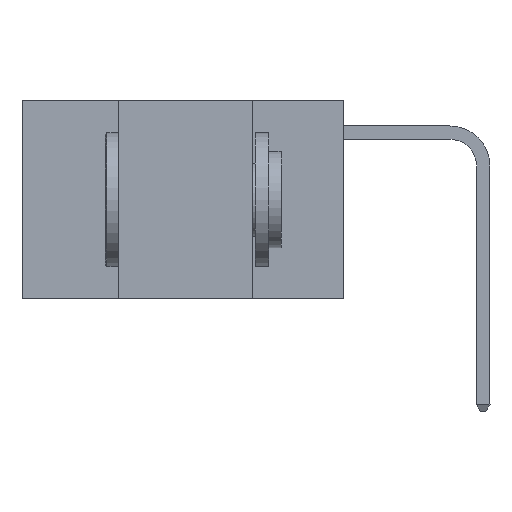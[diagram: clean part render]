
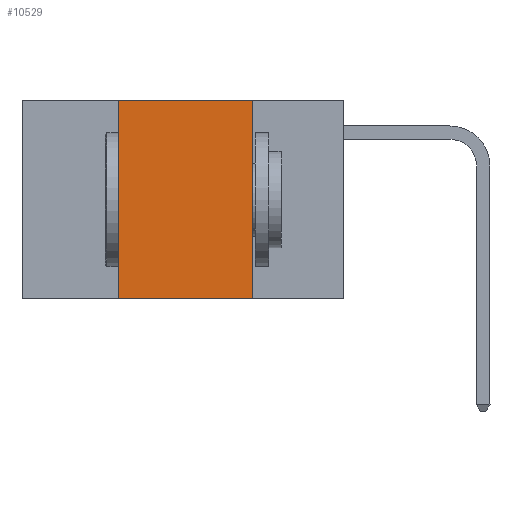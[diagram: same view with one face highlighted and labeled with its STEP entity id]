
A CAD part, left-side view. The second image highlights one B-rep face of the part: STEP entity #10529.
In plain terms, the highlighted planar face has unit normal (-1, 0, 0).
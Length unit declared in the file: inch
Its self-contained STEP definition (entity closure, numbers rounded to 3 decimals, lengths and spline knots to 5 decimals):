
#211 = CARTESIAN_POINT ( 'NONE',  ( 0., 0.42, -0.37 ) ) ;
#345 = PLANE ( 'NONE',  #6975 ) ;
#866 = CARTESIAN_POINT ( 'NONE',  ( 0., 0.17, -0.37 ) ) ;
#895 = VECTOR ( 'NONE', #1510, 39.37008 ) ;
#990 = ORIENTED_EDGE ( 'NONE', *, *, #8461, .F. ) ;
#1510 = DIRECTION ( 'NONE',  ( 0., 0., 1. ) ) ;
#1576 = EDGE_CURVE ( 'NONE', #8686, #7853, #7452, .T. ) ;
#1578 = DIRECTION ( 'NONE',  ( 0., 0., -1. ) ) ;
#1854 = VECTOR ( 'NONE', #11834, 39.37008 ) ;
#2192 = LINE ( 'NONE', #7042, #10957 ) ;
#3244 = FACE_OUTER_BOUND ( 'NONE', #6605, .T. ) ;
#4313 = ORIENTED_EDGE ( 'NONE', *, *, #9309, .T. ) ;
#4611 = ORIENTED_EDGE ( 'NONE', *, *, #1576, .F. ) ;
#5503 = VERTEX_POINT ( 'NONE', #866 ) ;
#6434 = DIRECTION ( 'NONE',  ( 0., 0., -1. ) ) ;
#6499 = LINE ( 'NONE', #10439, #10094 ) ;
#6605 = EDGE_LOOP ( 'NONE', ( #990, #7960, #4611, #4313 ) ) ;
#6975 = AXIS2_PLACEMENT_3D ( 'NONE', #9338, #9401, #6434 ) ;
#7042 = CARTESIAN_POINT ( 'NONE',  ( 0., 0.6, 0. ) ) ;
#7452 = LINE ( 'NONE', #10370, #895 ) ;
#7853 = VERTEX_POINT ( 'NONE', #9164 ) ;
#7879 = CARTESIAN_POINT ( 'NONE',  ( 0., 0.6, -0.37 ) ) ;
#7960 = ORIENTED_EDGE ( 'NONE', *, *, #11974, .F. ) ;
#8461 = EDGE_CURVE ( 'NONE', #9494, #5503, #6499, .T. ) ;
#8686 = VERTEX_POINT ( 'NONE', #211 ) ;
#9164 = CARTESIAN_POINT ( 'NONE',  ( 0., 0.42, 0. ) ) ;
#9309 = EDGE_CURVE ( 'NONE', #8686, #5503, #11708, .T. ) ;
#9338 = CARTESIAN_POINT ( 'NONE',  ( 0., 0.6, 0. ) ) ;
#9401 = DIRECTION ( 'NONE',  ( 1., 0., 0. ) ) ;
#9494 = VERTEX_POINT ( 'NONE', #11507 ) ;
#10094 = VECTOR ( 'NONE', #1578, 39.37008 ) ;
#10370 = CARTESIAN_POINT ( 'NONE',  ( 0., 0.42, 0. ) ) ;
#10439 = CARTESIAN_POINT ( 'NONE',  ( 0., 0.17, 0. ) ) ;
#10529 = ADVANCED_FACE ( 'NONE', ( #3244 ), #345, .F. ) ;
#10957 = VECTOR ( 'NONE', #11005, 39.37008 ) ;
#11005 = DIRECTION ( 'NONE',  ( 0., -1., 0. ) ) ;
#11507 = CARTESIAN_POINT ( 'NONE',  ( 0., 0.17, 0. ) ) ;
#11708 = LINE ( 'NONE', #7879, #1854 ) ;
#11834 = DIRECTION ( 'NONE',  ( 0., -1., 0. ) ) ;
#11974 = EDGE_CURVE ( 'NONE', #7853, #9494, #2192, .T. ) ;
